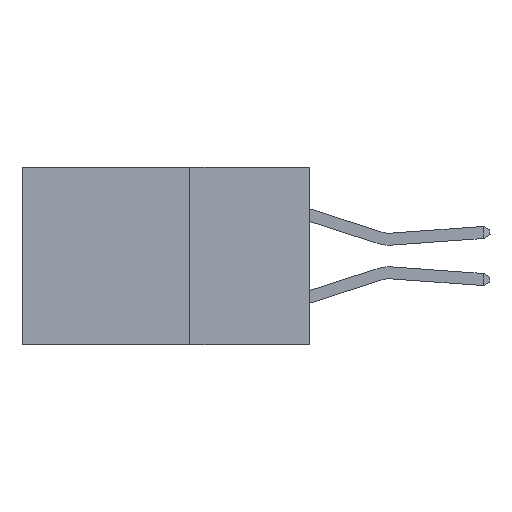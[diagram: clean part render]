
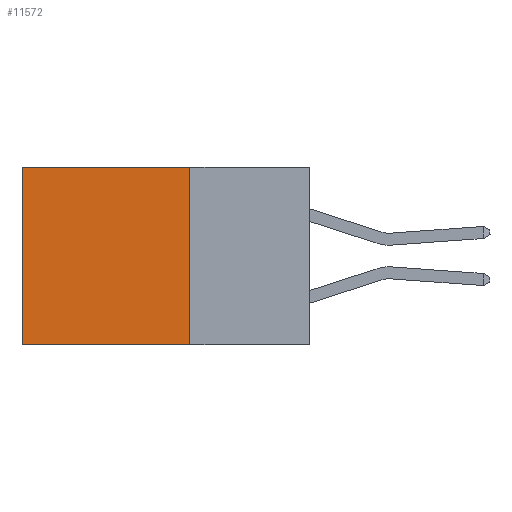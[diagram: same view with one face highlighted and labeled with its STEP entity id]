
A CAD part, left-side view. The second image highlights one B-rep face of the part: STEP entity #11572.
In plain terms, the highlighted planar face has unit normal (-1, 0, 0).
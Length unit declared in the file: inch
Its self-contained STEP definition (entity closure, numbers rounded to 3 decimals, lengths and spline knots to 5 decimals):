
#591 = CARTESIAN_POINT ( 'NONE',  ( 0.2615, 0.25, -0.37 ) ) ;
#705 = LINE ( 'NONE', #591, #11443 ) ;
#1091 = ORIENTED_EDGE ( 'NONE', *, *, #14748, .F. ) ;
#1914 = LINE ( 'NONE', #18099, #3840 ) ;
#2181 = CARTESIAN_POINT ( 'NONE',  ( 0.2615, 0.25, -0.37 ) ) ;
#3828 = VECTOR ( 'NONE', #16362, 39.37008 ) ;
#3840 = VECTOR ( 'NONE', #21363, 39.37008 ) ;
#4160 = EDGE_LOOP ( 'NONE', ( #16705, #18032, #1091, #7932 ) ) ;
#4497 = VERTEX_POINT ( 'NONE', #12573 ) ;
#5559 = CARTESIAN_POINT ( 'NONE',  ( 0.2615, 0.25, -0.37 ) ) ;
#5611 = DIRECTION ( 'NONE',  ( 0., 0., -1. ) ) ;
#6982 = PLANE ( 'NONE',  #15849 ) ;
#7672 = LINE ( 'NONE', #15941, #15738 ) ;
#7932 = ORIENTED_EDGE ( 'NONE', *, *, #17005, .T. ) ;
#8800 = FACE_OUTER_BOUND ( 'NONE', #4160, .T. ) ;
#11443 = VECTOR ( 'NONE', #17221, 39.37008 ) ;
#11572 = ADVANCED_FACE ( 'NONE', ( #8800 ), #6982, .F. ) ;
#12573 = CARTESIAN_POINT ( 'NONE',  ( 0.2615, 0.6, -0.37 ) ) ;
#12867 = CARTESIAN_POINT ( 'NONE',  ( 0.2615, 0.6, 0. ) ) ;
#13604 = DIRECTION ( 'NONE',  ( 0., 0., -1. ) ) ;
#14748 = EDGE_CURVE ( 'NONE', #18111, #21332, #705, .T. ) ;
#14905 = CARTESIAN_POINT ( 'NONE',  ( 0.2615, 0.25, 0. ) ) ;
#15738 = VECTOR ( 'NONE', #5611, 39.37008 ) ;
#15849 = AXIS2_PLACEMENT_3D ( 'NONE', #5559, #17402, #13604 ) ;
#15941 = CARTESIAN_POINT ( 'NONE',  ( 0.2615, 0.6, -0.37 ) ) ;
#16362 = DIRECTION ( 'NONE',  ( 0., 1., 0. ) ) ;
#16705 = ORIENTED_EDGE ( 'NONE', *, *, #18885, .T. ) ;
#17005 = EDGE_CURVE ( 'NONE', #18111, #18326, #20944, .T. ) ;
#17221 = DIRECTION ( 'NONE',  ( 0., 0., -1. ) ) ;
#17244 = EDGE_CURVE ( 'NONE', #21332, #4497, #1914, .T. ) ;
#17402 = DIRECTION ( 'NONE',  ( 1., 0., 0. ) ) ;
#18032 = ORIENTED_EDGE ( 'NONE', *, *, #17244, .F. ) ;
#18099 = CARTESIAN_POINT ( 'NONE',  ( 0.2615, 0.25, -0.37 ) ) ;
#18111 = VERTEX_POINT ( 'NONE', #14905 ) ;
#18326 = VERTEX_POINT ( 'NONE', #12867 ) ;
#18885 = EDGE_CURVE ( 'NONE', #18326, #4497, #7672, .T. ) ;
#20944 = LINE ( 'NONE', #21050, #3828 ) ;
#21050 = CARTESIAN_POINT ( 'NONE',  ( 0.2615, 0.25, 0. ) ) ;
#21332 = VERTEX_POINT ( 'NONE', #2181 ) ;
#21363 = DIRECTION ( 'NONE',  ( 0., 1., 0. ) ) ;
